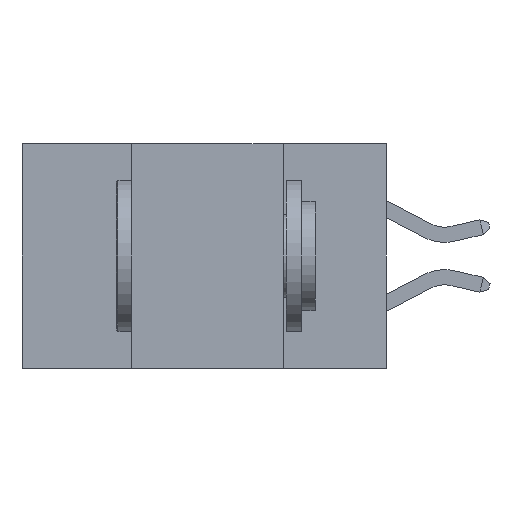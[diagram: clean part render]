
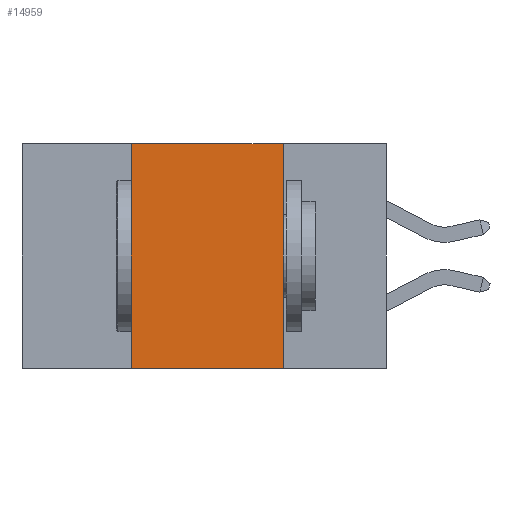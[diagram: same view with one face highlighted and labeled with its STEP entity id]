
A CAD part, left-side view. The second image highlights one B-rep face of the part: STEP entity #14959.
In plain terms, the highlighted planar face has unit normal (-1, 0, 0).
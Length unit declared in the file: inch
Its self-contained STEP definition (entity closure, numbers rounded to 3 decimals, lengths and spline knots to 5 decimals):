
#342 = EDGE_CURVE ( 'NONE', #2419, #12756, #12829, .T. ) ;
#487 = VECTOR ( 'NONE', #14398, 39.37008 ) ;
#2037 = EDGE_CURVE ( 'NONE', #11944, #19058, #7799, .T. ) ;
#2419 = VERTEX_POINT ( 'NONE', #15938 ) ;
#2676 = CARTESIAN_POINT ( 'NONE',  ( 0., 0.6, -0.37 ) ) ;
#4299 = CARTESIAN_POINT ( 'NONE',  ( 0., 0.6, 0. ) ) ;
#5420 = AXIS2_PLACEMENT_3D ( 'NONE', #4299, #5857, #18773 ) ;
#5520 = EDGE_CURVE ( 'NONE', #19058, #12756, #7374, .T. ) ;
#5857 = DIRECTION ( 'NONE',  ( 1., 0., 0. ) ) ;
#6237 = CARTESIAN_POINT ( 'NONE',  ( 0., 0.17, 0. ) ) ;
#7006 = CARTESIAN_POINT ( 'NONE',  ( 0., 0.6, 0. ) ) ;
#7289 = VECTOR ( 'NONE', #19441, 39.37008 ) ;
#7374 = LINE ( 'NONE', #6237, #12229 ) ;
#7472 = EDGE_LOOP ( 'NONE', ( #15017, #12970, #16479, #18138 ) ) ;
#7799 = LINE ( 'NONE', #7006, #7289 ) ;
#8162 = VECTOR ( 'NONE', #19405, 39.37008 ) ;
#8839 = CARTESIAN_POINT ( 'NONE',  ( 0., 0.42, 0. ) ) ;
#10444 = EDGE_CURVE ( 'NONE', #2419, #11944, #19775, .T. ) ;
#10981 = CARTESIAN_POINT ( 'NONE',  ( 0., 0.17, -0.37 ) ) ;
#11944 = VERTEX_POINT ( 'NONE', #12955 ) ;
#12229 = VECTOR ( 'NONE', #17068, 39.37008 ) ;
#12559 = FACE_OUTER_BOUND ( 'NONE', #7472, .T. ) ;
#12756 = VERTEX_POINT ( 'NONE', #10981 ) ;
#12829 = LINE ( 'NONE', #2676, #487 ) ;
#12955 = CARTESIAN_POINT ( 'NONE',  ( 0., 0.42, 0. ) ) ;
#12970 = ORIENTED_EDGE ( 'NONE', *, *, #2037, .F. ) ;
#14398 = DIRECTION ( 'NONE',  ( 0., -1., 0. ) ) ;
#14959 = ADVANCED_FACE ( 'NONE', ( #12559 ), #16614, .F. ) ;
#15017 = ORIENTED_EDGE ( 'NONE', *, *, #5520, .F. ) ;
#15869 = CARTESIAN_POINT ( 'NONE',  ( 0., 0.17, 0. ) ) ;
#15938 = CARTESIAN_POINT ( 'NONE',  ( 0., 0.42, -0.37 ) ) ;
#16479 = ORIENTED_EDGE ( 'NONE', *, *, #10444, .F. ) ;
#16614 = PLANE ( 'NONE',  #5420 ) ;
#17068 = DIRECTION ( 'NONE',  ( 0., 0., -1. ) ) ;
#18138 = ORIENTED_EDGE ( 'NONE', *, *, #342, .T. ) ;
#18773 = DIRECTION ( 'NONE',  ( 0., 0., -1. ) ) ;
#19058 = VERTEX_POINT ( 'NONE', #15869 ) ;
#19405 = DIRECTION ( 'NONE',  ( 0., 0., 1. ) ) ;
#19441 = DIRECTION ( 'NONE',  ( 0., -1., 0. ) ) ;
#19775 = LINE ( 'NONE', #8839, #8162 ) ;
